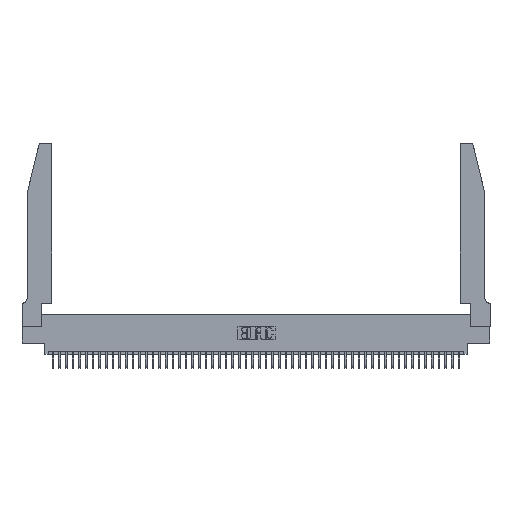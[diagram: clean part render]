
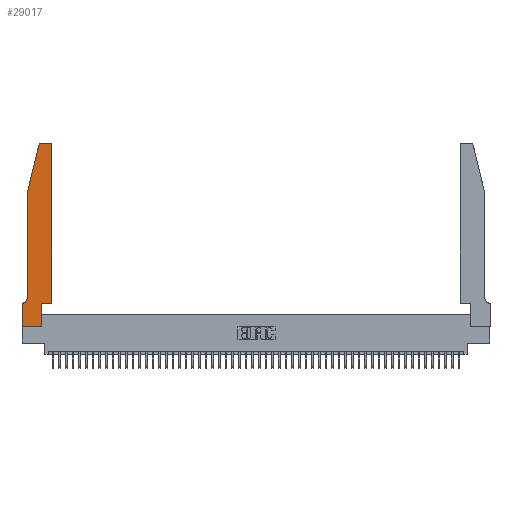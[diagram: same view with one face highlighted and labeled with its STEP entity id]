
A CAD part, top view. The second image highlights one B-rep face of the part: STEP entity #29017.
In plain terms, the highlighted planar face has unit normal (0, 0, 1).
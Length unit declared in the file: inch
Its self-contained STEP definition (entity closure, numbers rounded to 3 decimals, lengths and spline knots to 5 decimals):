
#516 = CARTESIAN_POINT ( 'NONE',  ( 0., 0., 0.37 ) ) ;
#1076 = CARTESIAN_POINT ( 'NONE',  ( 0.0755, 2., 0.37 ) ) ;
#1155 = EDGE_CURVE ( 'NONE', #36250, #40013, #20977, .T. ) ;
#2146 = CARTESIAN_POINT ( 'NONE',  ( 0.0755, 0.42, 0.37 ) ) ;
#2688 = AXIS2_PLACEMENT_3D ( 'NONE', #34383, #6730, #47110 ) ;
#3357 = ORIENTED_EDGE ( 'NONE', *, *, #23154, .T. ) ;
#4250 = VERTEX_POINT ( 'NONE', #46024 ) ;
#4432 = DIRECTION ( 'NONE',  ( -0.239, -0.971, 0. ) ) ;
#4650 = AXIS2_PLACEMENT_3D ( 'NONE', #45620, #21374, #49709 ) ;
#5384 = VERTEX_POINT ( 'NONE', #22222 ) ;
#5785 = ORIENTED_EDGE ( 'NONE', *, *, #49167, .T. ) ;
#6050 = LINE ( 'NONE', #35382, #26957 ) ;
#6730 = DIRECTION ( 'NONE',  ( 0., 0., 1. ) ) ;
#10314 = VERTEX_POINT ( 'NONE', #46439 ) ;
#10643 = FACE_OUTER_BOUND ( 'NONE', #11172, .T. ) ;
#11172 = EDGE_LOOP ( 'NONE', ( #28083, #47761, #17215, #12749, #29153, #50339, #3357, #18023, #34442, #18685, #43647, #5785 ) ) ;
#11739 = LINE ( 'NONE', #516, #16216 ) ;
#12749 = ORIENTED_EDGE ( 'NONE', *, *, #30640, .T. ) ;
#12825 = DIRECTION ( 'NONE',  ( 0., -1., 0. ) ) ;
#13201 = LINE ( 'NONE', #16020, #51189 ) ;
#13332 = VERTEX_POINT ( 'NONE', #32047 ) ;
#13432 = CARTESIAN_POINT ( 'NONE',  ( 0., 0.35, 0.37 ) ) ;
#13560 = CARTESIAN_POINT ( 'NONE',  ( 0.2865, 0.35, 0.37 ) ) ;
#14100 = CARTESIAN_POINT ( 'NONE',  ( 0.4205, 2.75, 0.37 ) ) ;
#14469 = LINE ( 'NONE', #13560, #37212 ) ;
#15705 = LINE ( 'NONE', #26449, #50564 ) ;
#15886 = CARTESIAN_POINT ( 'NONE',  ( 0.25487, 2.72718, 0.37 ) ) ;
#15960 = CARTESIAN_POINT ( 'NONE',  ( 0.0755, 2., 0.37 ) ) ;
#16020 = CARTESIAN_POINT ( 'NONE',  ( 0.0755, 2., 0.37 ) ) ;
#16095 = EDGE_CURVE ( 'NONE', #48415, #42326, #17317, .T. ) ;
#16216 = VECTOR ( 'NONE', #12825, 39.37008 ) ;
#17215 = ORIENTED_EDGE ( 'NONE', *, *, #46226, .T. ) ;
#17317 = CIRCLE ( 'NONE', #22819, 0.07 ) ;
#17630 = DIRECTION ( 'NONE',  ( 0., 1., 0. ) ) ;
#18023 = ORIENTED_EDGE ( 'NONE', *, *, #39450, .T. ) ;
#18685 = ORIENTED_EDGE ( 'NONE', *, *, #44583, .T. ) ;
#18756 = DIRECTION ( 'NONE',  ( -1., 0., 0. ) ) ;
#18942 = VERTEX_POINT ( 'NONE', #46515 ) ;
#18948 = LINE ( 'NONE', #50419, #23324 ) ;
#19595 = EDGE_CURVE ( 'NONE', #38477, #36250, #36729, .T. ) ;
#20758 = EDGE_CURVE ( 'NONE', #42326, #10314, #41705, .T. ) ;
#20789 = CARTESIAN_POINT ( 'NONE',  ( 0.284, 2.75, 0.37 ) ) ;
#20952 = DIRECTION ( 'NONE',  ( 0., 0., -1. ) ) ;
#20977 = CIRCLE ( 'NONE', #2688, 0.03 ) ;
#21374 = DIRECTION ( 'NONE',  ( 0., 0., 1. ) ) ;
#22222 = CARTESIAN_POINT ( 'NONE',  ( 0.2865, 0., 0.37 ) ) ;
#22819 = AXIS2_PLACEMENT_3D ( 'NONE', #49293, #20952, #29479 ) ;
#23092 = VERTEX_POINT ( 'NONE', #1076 ) ;
#23154 = EDGE_CURVE ( 'NONE', #10314, #13332, #11739, .T. ) ;
#23324 = VECTOR ( 'NONE', #30087, 39.37008 ) ;
#23702 = DIRECTION ( 'NONE',  ( 1., 0., 0. ) ) ;
#23725 = DIRECTION ( 'NONE',  ( 0., -1., 0. ) ) ;
#26449 = CARTESIAN_POINT ( 'NONE',  ( 0.4505, 0.35, 0.37 ) ) ;
#26957 = VECTOR ( 'NONE', #23702, 39.37008 ) ;
#27471 = CIRCLE ( 'NONE', #4650, 0.03 ) ;
#28053 = VERTEX_POINT ( 'NONE', #31214 ) ;
#28083 = ORIENTED_EDGE ( 'NONE', *, *, #19595, .T. ) ;
#29017 = ADVANCED_FACE ( 'NONE', ( #10643 ), #34113, .T. ) ;
#29153 = ORIENTED_EDGE ( 'NONE', *, *, #16095, .T. ) ;
#29479 = DIRECTION ( 'NONE',  ( -1., 0., 0. ) ) ;
#30087 = DIRECTION ( 'NONE',  ( 0., 1., 0. ) ) ;
#30640 = EDGE_CURVE ( 'NONE', #23092, #48415, #42201, .T. ) ;
#30978 = VECTOR ( 'NONE', #18756, 39.37008 ) ;
#31214 = CARTESIAN_POINT ( 'NONE',  ( 0.4505, 2.72, 0.37 ) ) ;
#32047 = CARTESIAN_POINT ( 'NONE',  ( 0., 0., 0.37 ) ) ;
#32972 = VECTOR ( 'NONE', #52360, 39.37008 ) ;
#34113 = PLANE ( 'NONE',  #48943 ) ;
#34383 = CARTESIAN_POINT ( 'NONE',  ( 0.284, 2.72, 0.37 ) ) ;
#34442 = ORIENTED_EDGE ( 'NONE', *, *, #36398, .T. ) ;
#35382 = CARTESIAN_POINT ( 'NONE',  ( 0., 0., 0.37 ) ) ;
#36250 = VERTEX_POINT ( 'NONE', #20789 ) ;
#36398 = EDGE_CURVE ( 'NONE', #5384, #18942, #14469, .T. ) ;
#36729 = LINE ( 'NONE', #52527, #32972 ) ;
#37212 = VECTOR ( 'NONE', #17630, 39.37008 ) ;
#37655 = CARTESIAN_POINT ( 'NONE',  ( 0.0755, 0.35, 0.37 ) ) ;
#38477 = VERTEX_POINT ( 'NONE', #14100 ) ;
#38807 = DIRECTION ( 'NONE',  ( 1., 0., 0. ) ) ;
#39450 = EDGE_CURVE ( 'NONE', #13332, #5384, #6050, .T. ) ;
#39635 = VECTOR ( 'NONE', #23725, 39.37008 ) ;
#40013 = VERTEX_POINT ( 'NONE', #15886 ) ;
#41705 = LINE ( 'NONE', #37655, #30978 ) ;
#42201 = LINE ( 'NONE', #15960, #39635 ) ;
#42247 = DIRECTION ( 'NONE',  ( 0., 0., 1. ) ) ;
#42326 = VERTEX_POINT ( 'NONE', #44519 ) ;
#43647 = ORIENTED_EDGE ( 'NONE', *, *, #45723, .T. ) ;
#44519 = CARTESIAN_POINT ( 'NONE',  ( 0.0055, 0.35, 0.37 ) ) ;
#44583 = EDGE_CURVE ( 'NONE', #18942, #4250, #15705, .T. ) ;
#45620 = CARTESIAN_POINT ( 'NONE',  ( 0.4205, 2.72, 0.37 ) ) ;
#45723 = EDGE_CURVE ( 'NONE', #4250, #28053, #18948, .T. ) ;
#46024 = CARTESIAN_POINT ( 'NONE',  ( 0.4505, 0.35, 0.37 ) ) ;
#46226 = EDGE_CURVE ( 'NONE', #40013, #23092, #13201, .T. ) ;
#46325 = DIRECTION ( 'NONE',  ( 1., 0., 0. ) ) ;
#46439 = CARTESIAN_POINT ( 'NONE',  ( 0., 0.35, 0.37 ) ) ;
#46515 = CARTESIAN_POINT ( 'NONE',  ( 0.2865, 0.35, 0.37 ) ) ;
#47110 = DIRECTION ( 'NONE',  ( 1., 0., 0. ) ) ;
#47761 = ORIENTED_EDGE ( 'NONE', *, *, #1155, .T. ) ;
#48415 = VERTEX_POINT ( 'NONE', #2146 ) ;
#48943 = AXIS2_PLACEMENT_3D ( 'NONE', #13432, #42247, #46325 ) ;
#49167 = EDGE_CURVE ( 'NONE', #28053, #38477, #27471, .T. ) ;
#49293 = CARTESIAN_POINT ( 'NONE',  ( 0.0055, 0.42, 0.37 ) ) ;
#49709 = DIRECTION ( 'NONE',  ( 1., 0., 0. ) ) ;
#50339 = ORIENTED_EDGE ( 'NONE', *, *, #20758, .T. ) ;
#50419 = CARTESIAN_POINT ( 'NONE',  ( 0.4505, 0.35, 0.37 ) ) ;
#50564 = VECTOR ( 'NONE', #38807, 39.37008 ) ;
#51189 = VECTOR ( 'NONE', #4432, 39.37008 ) ;
#52360 = DIRECTION ( 'NONE',  ( -1., 0., 0. ) ) ;
#52527 = CARTESIAN_POINT ( 'NONE',  ( 0.2605, 2.75, 0.37 ) ) ;
